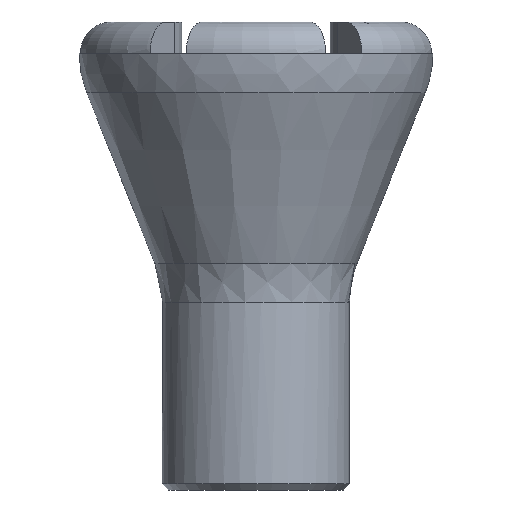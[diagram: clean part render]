
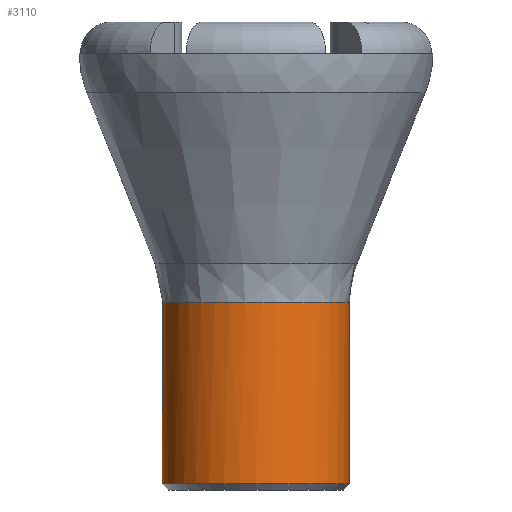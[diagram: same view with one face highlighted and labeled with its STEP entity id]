
A CAD part, front view. The second image highlights one B-rep face of the part: STEP entity #3110.
In plain terms, the highlighted cylindrical face has radius 9 mm (diameter 18 mm), a full revolution.
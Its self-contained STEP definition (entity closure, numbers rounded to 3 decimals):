
#2977 = ( BOUNDED_SURFACE() B_SPLINE_SURFACE(2,14,(
    (#2978,#2979,#2980,#2981,#2982,#2983,#2984,#2985,#2986,#2987,#2988
      ,#2989,#2990,#2991,#2992)
    ,(#2993,#2994,#2995,#2996,#2997,#2998,#2999,#3000,#3001,#3002,#3003
      ,#3004,#3005,#3006,#3007)
    ,(#3008,#3009,#3010,#3011,#3012,#3013,#3014,#3015,#3016,#3017,#3018
      ,#3019,#3020,#3021,#3022
)),.UNSPECIFIED.,.F.,.T.,.F.) B_SPLINE_SURFACE_WITH_KNOTS((3,3),(15,15),
  (0.,56.549),(0.,56.549),.PIECEWISE_BEZIER_KNOTS.) 
GEOMETRIC_REPRESENTATION_ITEM() RATIONAL_B_SPLINE_SURFACE((
    (1.,1.,1.,1.,1.
      ,1.,1.,1.,1.
      ,1.,1.,1.,1.
      ,1.,1.)
    ,(0.982,0.982,0.982,0.982
      ,0.982,0.982,0.982,0.982
      ,0.982,0.982,0.982,0.982
      ,0.982,0.982,0.982)
    ,(1.,1.,1.,1.,1.
      ,1.,1.,1.,1.
      ,1.,1.,1.,1.
,1.,1.))) REPRESENTATION_ITEM('') SURFACE() );
#2978 = CARTESIAN_POINT('',(9.715,0.,51.788));
#2979 = CARTESIAN_POINT('',(9.715,4.297,51.788
    ));
#2980 = CARTESIAN_POINT('',(7.669,8.686,
    51.788));
#2981 = CARTESIAN_POINT('',(3.431,12.022,
    51.788));
#2982 = CARTESIAN_POINT('',(-2.348,13.119,
    51.788));
#2983 = CARTESIAN_POINT('',(-8.335,10.948,
    51.788));
#2984 = CARTESIAN_POINT('',(-12.351,6.649,
    51.788));
#2985 = CARTESIAN_POINT('',(-14.892,0.,51.788)
  );
#2986 = CARTESIAN_POINT('',(-12.351,-6.649,
    51.788));
#2987 = CARTESIAN_POINT('',(-8.335,-10.948,
    51.788));
#2988 = CARTESIAN_POINT('',(-2.348,-13.119,
    51.788));
#2989 = CARTESIAN_POINT('',(3.431,-12.022,
    51.788));
#2990 = CARTESIAN_POINT('',(7.669,-8.686,
    51.788));
#2991 = CARTESIAN_POINT('',(9.715,-4.297,
    51.788));
#2992 = CARTESIAN_POINT('',(9.715,0.,51.788));
#2993 = CARTESIAN_POINT('',(9.,0.,50.));
#2994 = CARTESIAN_POINT('',(9.,3.981,50.));
#2995 = CARTESIAN_POINT('',(7.104,8.046,50.));
#2996 = CARTESIAN_POINT('',(3.179,11.137,50.));
#2997 = CARTESIAN_POINT('',(-2.175,12.153,50.));
#2998 = CARTESIAN_POINT('',(-7.721,10.142,
    50.));
#2999 = CARTESIAN_POINT('',(-11.442,6.16,
    50.));
#3000 = CARTESIAN_POINT('',(-13.795,0.,50.)
  );
#3001 = CARTESIAN_POINT('',(-11.442,-6.16,
    50.));
#3002 = CARTESIAN_POINT('',(-7.721,-10.142,
    50.));
#3003 = CARTESIAN_POINT('',(-2.175,-12.153,50.));
#3004 = CARTESIAN_POINT('',(3.179,-11.137,50.));
#3005 = CARTESIAN_POINT('',(7.104,-8.046,50.));
#3006 = CARTESIAN_POINT('',(9.,-3.981,50.));
#3007 = CARTESIAN_POINT('',(9.,0.,50.));
#3008 = CARTESIAN_POINT('',(9.,0.,48.074));
#3009 = CARTESIAN_POINT('',(9.,3.981,
    48.074));
#3010 = CARTESIAN_POINT('',(7.104,8.046,
    48.074));
#3011 = CARTESIAN_POINT('',(3.179,11.137,
    48.074));
#3012 = CARTESIAN_POINT('',(-2.175,12.153,
    48.074));
#3013 = CARTESIAN_POINT('',(-7.721,10.142,
    48.074));
#3014 = CARTESIAN_POINT('',(-11.442,6.16,
    48.074));
#3015 = CARTESIAN_POINT('',(-13.795,0.,48.074
    ));
#3016 = CARTESIAN_POINT('',(-11.442,-6.16,
    48.074));
#3017 = CARTESIAN_POINT('',(-7.721,-10.142,
    48.074));
#3018 = CARTESIAN_POINT('',(-2.175,-12.153,
    48.074));
#3019 = CARTESIAN_POINT('',(3.179,-11.137,
    48.074));
#3020 = CARTESIAN_POINT('',(7.104,-8.046,
    48.074));
#3021 = CARTESIAN_POINT('',(9.,-3.981,
    48.074));
#3022 = CARTESIAN_POINT('',(9.,0.,48.074));
#3034 = VERTEX_POINT('',#3035);
#3035 = CARTESIAN_POINT('',(9.,0.,48.074));
#3054 = EDGE_CURVE('',#3034,#3034,#3055,.T.);
#3055 = SURFACE_CURVE('',#3056,(#3072,#3079),.PCURVE_S1.);
#3056 = ( BOUNDED_CURVE() B_SPLINE_CURVE(14,(#3057,#3058,#3059,#3060,
    #3061,#3062,#3063,#3064,#3065,#3066,#3067,#3068,#3069,#3070,#3071),
.UNSPECIFIED.,.T.,.F.) B_SPLINE_CURVE_WITH_KNOTS((15,15),(0.,
56.549),.PIECEWISE_BEZIER_KNOTS.) CURVE() 
GEOMETRIC_REPRESENTATION_ITEM() RATIONAL_B_SPLINE_CURVE((1.,
    1.,1.,1.,1.,
    1.,1.,1.,1.,
    1.,1.,1.,1.,
1.,1.)) REPRESENTATION_ITEM('') );
#3057 = CARTESIAN_POINT('',(9.,0.,48.074));
#3058 = CARTESIAN_POINT('',(9.,3.981,
    48.074));
#3059 = CARTESIAN_POINT('',(7.104,8.046,
    48.074));
#3060 = CARTESIAN_POINT('',(3.179,11.137,
    48.074));
#3061 = CARTESIAN_POINT('',(-2.175,12.153,
    48.074));
#3062 = CARTESIAN_POINT('',(-7.721,10.142,
    48.074));
#3063 = CARTESIAN_POINT('',(-11.442,6.16,
    48.074));
#3064 = CARTESIAN_POINT('',(-13.795,0.,48.074
    ));
#3065 = CARTESIAN_POINT('',(-11.442,-6.16,
    48.074));
#3066 = CARTESIAN_POINT('',(-7.721,-10.142,
    48.074));
#3067 = CARTESIAN_POINT('',(-2.175,-12.153,
    48.074));
#3068 = CARTESIAN_POINT('',(3.179,-11.137,
    48.074));
#3069 = CARTESIAN_POINT('',(7.104,-8.046,
    48.074));
#3070 = CARTESIAN_POINT('',(9.,-3.981,
    48.074));
#3071 = CARTESIAN_POINT('',(9.,0.,48.074));
#3072 = PCURVE('',#2977,#3073);
#3073 = DEFINITIONAL_REPRESENTATION('',(#3074),#3078);
#3074 = LINE('',#3075,#3076);
#3075 = CARTESIAN_POINT('',(56.549,0.));
#3076 = VECTOR('',#3077,1.);
#3077 = DIRECTION('',(0.,1.));
#3078 = ( GEOMETRIC_REPRESENTATION_CONTEXT(2) 
PARAMETRIC_REPRESENTATION_CONTEXT() REPRESENTATION_CONTEXT('2D SPACE',''
  ) );
#3079 = PCURVE('',#3080,#3085);
#3080 = CYLINDRICAL_SURFACE('',#3081,9.);
#3081 = AXIS2_PLACEMENT_3D('',#3082,#3083,#3084);
#3082 = CARTESIAN_POINT('',(0.,0.,30.));
#3083 = DIRECTION('',(-0.,-0.,-1.));
#3084 = DIRECTION('',(1.,0.,0.));
#3085 = DEFINITIONAL_REPRESENTATION('',(#3086),#3107);
#3086 = B_SPLINE_CURVE_WITH_KNOTS('',10,(#3087,#3088,#3089,#3090,#3091,
    #3092,#3093,#3094,#3095,#3096,#3097,#3098,#3099,#3100,#3101,#3102,
    #3103,#3104,#3105,#3106),.UNSPECIFIED.,.F.,.F.,(11,9,11),(0.,
    28.274,56.549),.UNSPECIFIED.);
#3087 = CARTESIAN_POINT('',(0.,-18.074));
#3088 = CARTESIAN_POINT('',(-0.31,-18.074));
#3089 = CARTESIAN_POINT('',(-0.624,-18.074));
#3090 = CARTESIAN_POINT('',(-0.94,-18.074));
#3091 = CARTESIAN_POINT('',(-1.256,-18.074));
#3092 = CARTESIAN_POINT('',(-1.57,-18.074));
#3093 = CARTESIAN_POINT('',(-1.885,-18.074));
#3094 = CARTESIAN_POINT('',(-2.199,-18.074));
#3095 = CARTESIAN_POINT('',(-2.513,-18.074));
#3096 = CARTESIAN_POINT('',(-2.827,-18.074));
#3097 = CARTESIAN_POINT('',(-3.456,-18.074));
#3098 = CARTESIAN_POINT('',(-3.77,-18.074));
#3099 = CARTESIAN_POINT('',(-4.084,-18.074));
#3100 = CARTESIAN_POINT('',(-4.398,-18.074));
#3101 = CARTESIAN_POINT('',(-4.713,-18.074));
#3102 = CARTESIAN_POINT('',(-5.027,-18.074));
#3103 = CARTESIAN_POINT('',(-5.343,-18.074));
#3104 = CARTESIAN_POINT('',(-5.659,-18.074));
#3105 = CARTESIAN_POINT('',(-5.974,-18.074));
#3106 = CARTESIAN_POINT('',(-6.283,-18.074));
#3107 = ( GEOMETRIC_REPRESENTATION_CONTEXT(2) 
PARAMETRIC_REPRESENTATION_CONTEXT() REPRESENTATION_CONTEXT('2D SPACE',''
  ) );
#3110 = ADVANCED_FACE('',(#3111),#3080,.T.);
#3111 = FACE_BOUND('',#3112,.F.);
#3112 = EDGE_LOOP('',(#3113,#3136,#3137,#3138));
#3113 = ORIENTED_EDGE('',*,*,#3114,.T.);
#3114 = EDGE_CURVE('',#3115,#3034,#3117,.T.);
#3115 = VERTEX_POINT('',#3116);
#3116 = CARTESIAN_POINT('',(9.,0.,30.6));
#3117 = SEAM_CURVE('',#3118,(#3122,#3129),.PCURVE_S1.);
#3118 = LINE('',#3119,#3120);
#3119 = CARTESIAN_POINT('',(9.,0.,30.));
#3120 = VECTOR('',#3121,1.);
#3121 = DIRECTION('',(0.,0.,1.));
#3122 = PCURVE('',#3080,#3123);
#3123 = DEFINITIONAL_REPRESENTATION('',(#3124),#3128);
#3124 = LINE('',#3125,#3126);
#3125 = CARTESIAN_POINT('',(-0.,0.));
#3126 = VECTOR('',#3127,1.);
#3127 = DIRECTION('',(-0.,-1.));
#3128 = ( GEOMETRIC_REPRESENTATION_CONTEXT(2) 
PARAMETRIC_REPRESENTATION_CONTEXT() REPRESENTATION_CONTEXT('2D SPACE',''
  ) );
#3129 = PCURVE('',#3080,#3130);
#3130 = DEFINITIONAL_REPRESENTATION('',(#3131),#3135);
#3131 = LINE('',#3132,#3133);
#3132 = CARTESIAN_POINT('',(-6.283,0.));
#3133 = VECTOR('',#3134,1.);
#3134 = DIRECTION('',(-0.,-1.));
#3135 = ( GEOMETRIC_REPRESENTATION_CONTEXT(2) 
PARAMETRIC_REPRESENTATION_CONTEXT() REPRESENTATION_CONTEXT('2D SPACE',''
  ) );
#3136 = ORIENTED_EDGE('',*,*,#3054,.T.);
#3137 = ORIENTED_EDGE('',*,*,#3114,.F.);
#3138 = ORIENTED_EDGE('',*,*,#3139,.F.);
#3139 = EDGE_CURVE('',#3115,#3115,#3140,.T.);
#3140 = SURFACE_CURVE('',#3141,(#3146,#3153),.PCURVE_S1.);
#3141 = CIRCLE('',#3142,9.);
#3142 = AXIS2_PLACEMENT_3D('',#3143,#3144,#3145);
#3143 = CARTESIAN_POINT('',(0.,0.,30.6));
#3144 = DIRECTION('',(0.,0.,1.));
#3145 = DIRECTION('',(1.,0.,0.));
#3146 = PCURVE('',#3080,#3147);
#3147 = DEFINITIONAL_REPRESENTATION('',(#3148),#3152);
#3148 = LINE('',#3149,#3150);
#3149 = CARTESIAN_POINT('',(-0.,-0.6));
#3150 = VECTOR('',#3151,1.);
#3151 = DIRECTION('',(-1.,0.));
#3152 = ( GEOMETRIC_REPRESENTATION_CONTEXT(2) 
PARAMETRIC_REPRESENTATION_CONTEXT() REPRESENTATION_CONTEXT('2D SPACE',''
  ) );
#3153 = PCURVE('',#3154,#3159);
#3154 = CONICAL_SURFACE('',#3155,9.,0.785);
#3155 = AXIS2_PLACEMENT_3D('',#3156,#3157,#3158);
#3156 = CARTESIAN_POINT('',(0.,0.,30.6));
#3157 = DIRECTION('',(0.,0.,1.));
#3158 = DIRECTION('',(1.,0.,0.));
#3159 = DEFINITIONAL_REPRESENTATION('',(#3160),#3164);
#3160 = LINE('',#3161,#3162);
#3161 = CARTESIAN_POINT('',(0.,-0.));
#3162 = VECTOR('',#3163,1.);
#3163 = DIRECTION('',(1.,-0.));
#3164 = ( GEOMETRIC_REPRESENTATION_CONTEXT(2) 
PARAMETRIC_REPRESENTATION_CONTEXT() REPRESENTATION_CONTEXT('2D SPACE',''
  ) );
